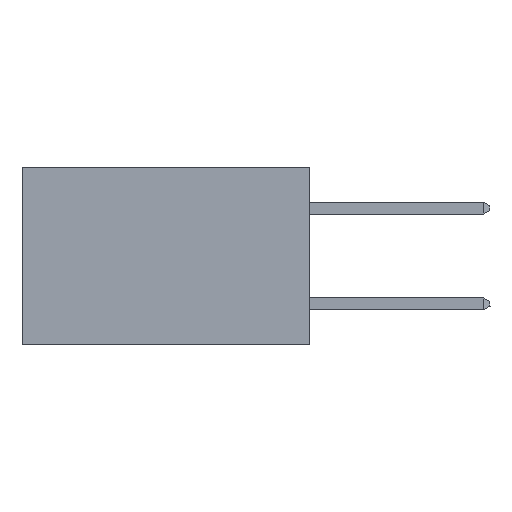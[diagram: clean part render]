
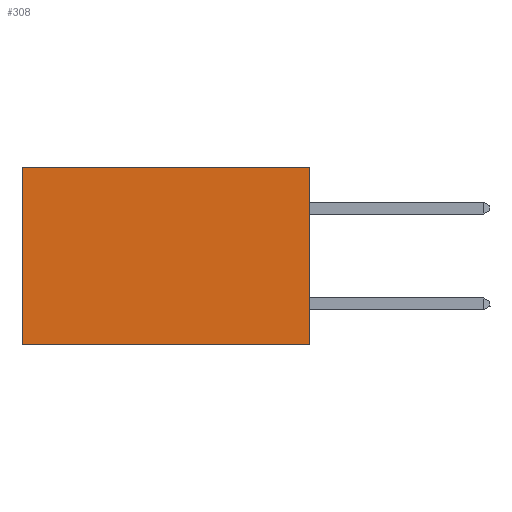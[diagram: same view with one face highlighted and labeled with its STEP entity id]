
A CAD part, left-side view. The second image highlights one B-rep face of the part: STEP entity #308.
In plain terms, the highlighted planar face has unit normal (-1, 0, 0).
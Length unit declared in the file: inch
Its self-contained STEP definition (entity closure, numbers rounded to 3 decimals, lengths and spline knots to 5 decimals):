
#227 = VECTOR ( 'NONE', #11101, 39.37008 ) ;
#308 = ADVANCED_FACE ( 'NONE', ( #10561 ), #8579, .F. ) ;
#502 = ORIENTED_EDGE ( 'NONE', *, *, #4956, .F. ) ;
#611 = ORIENTED_EDGE ( 'NONE', *, *, #11266, .F. ) ;
#624 = ORIENTED_EDGE ( 'NONE', *, *, #1166, .T. ) ;
#833 = VERTEX_POINT ( 'NONE', #5871 ) ;
#1017 = VECTOR ( 'NONE', #10812, 39.37008 ) ;
#1077 = VECTOR ( 'NONE', #1998, 39.37008 ) ;
#1166 = EDGE_CURVE ( 'NONE', #3138, #833, #11547, .T. ) ;
#1308 = DIRECTION ( 'NONE',  ( 0., 1., 0. ) ) ;
#1998 = DIRECTION ( 'NONE',  ( 0., 0., -1. ) ) ;
#2255 = CARTESIAN_POINT ( 'NONE',  ( 0.2875, 0.6, -0.37 ) ) ;
#2559 = ORIENTED_EDGE ( 'NONE', *, *, #5745, .T. ) ;
#2811 = EDGE_LOOP ( 'NONE', ( #2559, #502, #611, #624 ) ) ;
#3087 = LINE ( 'NONE', #11281, #227 ) ;
#3138 = VERTEX_POINT ( 'NONE', #5980 ) ;
#3770 = DIRECTION ( 'NONE',  ( 1., 0., 0. ) ) ;
#3875 = LINE ( 'NONE', #9300, #1077 ) ;
#4439 = VECTOR ( 'NONE', #1308, 39.37008 ) ;
#4956 = EDGE_CURVE ( 'NONE', #10560, #6238, #3087, .T. ) ;
#5265 = CARTESIAN_POINT ( 'NONE',  ( 0.2875, 0., 0. ) ) ;
#5745 = EDGE_CURVE ( 'NONE', #833, #6238, #3875, .T. ) ;
#5766 = CARTESIAN_POINT ( 'NONE',  ( 0.2875, 0., 0. ) ) ;
#5871 = CARTESIAN_POINT ( 'NONE',  ( 0.2875, 0.6, 0. ) ) ;
#5980 = CARTESIAN_POINT ( 'NONE',  ( 0.2875, 0., 0. ) ) ;
#6238 = VERTEX_POINT ( 'NONE', #2255 ) ;
#6769 = CARTESIAN_POINT ( 'NONE',  ( 0.2875, 0., -0.37 ) ) ;
#7412 = DIRECTION ( 'NONE',  ( 0., 0., -1. ) ) ;
#7619 = AXIS2_PLACEMENT_3D ( 'NONE', #5766, #3770, #7412 ) ;
#8579 = PLANE ( 'NONE',  #7619 ) ;
#9300 = CARTESIAN_POINT ( 'NONE',  ( 0.2875, 0.6, 0. ) ) ;
#10485 = CARTESIAN_POINT ( 'NONE',  ( 0.2875, 0., 0. ) ) ;
#10560 = VERTEX_POINT ( 'NONE', #6769 ) ;
#10561 = FACE_OUTER_BOUND ( 'NONE', #2811, .T. ) ;
#10696 = LINE ( 'NONE', #5265, #1017 ) ;
#10812 = DIRECTION ( 'NONE',  ( 0., 0., -1. ) ) ;
#11101 = DIRECTION ( 'NONE',  ( 0., 1., 0. ) ) ;
#11266 = EDGE_CURVE ( 'NONE', #3138, #10560, #10696, .T. ) ;
#11281 = CARTESIAN_POINT ( 'NONE',  ( 0.2875, 0., -0.37 ) ) ;
#11547 = LINE ( 'NONE', #10485, #4439 ) ;
